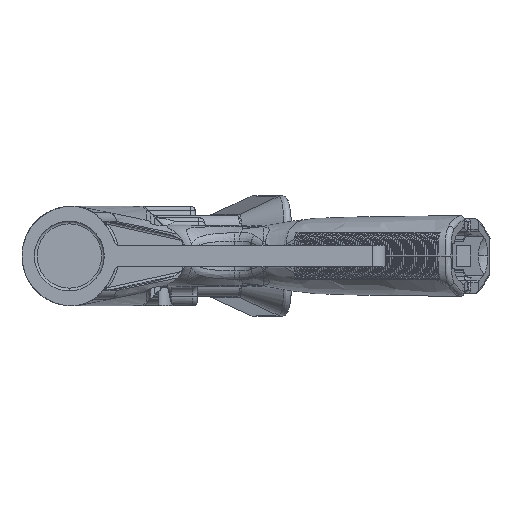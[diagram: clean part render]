
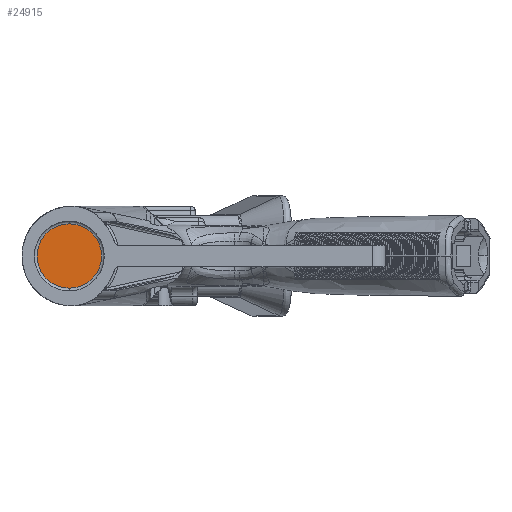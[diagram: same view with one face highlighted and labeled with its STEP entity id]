
A CAD part, left-side view. The second image highlights one B-rep face of the part: STEP entity #24915.
In plain terms, the highlighted planar face has unit normal (-1, 0, 0).
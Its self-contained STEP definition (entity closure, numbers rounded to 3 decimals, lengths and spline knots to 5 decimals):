
#762 = CIRCLE ( 'NONE', #21061, 0.47244 ) ;
#9850 = AXIS2_PLACEMENT_3D ( 'NONE', #50701, #78847, #23850 ) ;
#11358 = CIRCLE ( 'NONE', #9850, 0.47244 ) ;
#11780 = DIRECTION ( 'NONE',  ( 0., 0., 1. ) ) ;
#12661 = VERTEX_POINT ( 'NONE', #74836 ) ;
#18324 = EDGE_CURVE ( 'NONE', #82967, #12661, #11358, .T. ) ;
#21061 = AXIS2_PLACEMENT_3D ( 'NONE', #56639, #43883, #22078 ) ;
#22078 = DIRECTION ( 'NONE',  ( 0., 0., 1. ) ) ;
#23820 = ORIENTED_EDGE ( 'NONE', *, *, #65666, .T. ) ;
#23850 = DIRECTION ( 'NONE',  ( 0., 0., 1. ) ) ;
#24915 = ADVANCED_FACE ( 'NONE', ( #54492 ), #25848, .T. ) ;
#25848 = PLANE ( 'NONE',  #40679 ) ;
#39857 = EDGE_LOOP ( 'NONE', ( #60450, #23820 ) ) ;
#40679 = AXIS2_PLACEMENT_3D ( 'NONE', #46754, #80406, #11780 ) ;
#43883 = DIRECTION ( 'NONE',  ( -1., 0., 0. ) ) ;
#46754 = CARTESIAN_POINT ( 'NONE',  ( -14.68504, 0.87992, 0. ) ) ;
#50701 = CARTESIAN_POINT ( 'NONE',  ( -14.68504, 0.87992, 0. ) ) ;
#54492 = FACE_OUTER_BOUND ( 'NONE', #39857, .T. ) ;
#56639 = CARTESIAN_POINT ( 'NONE',  ( -14.68504, 0.87992, 0. ) ) ;
#60450 = ORIENTED_EDGE ( 'NONE', *, *, #18324, .T. ) ;
#65666 = EDGE_CURVE ( 'NONE', #12661, #82967, #762, .T. ) ;
#70736 = CARTESIAN_POINT ( 'NONE',  ( -14.68504, 0.87992, 0.47244 ) ) ;
#74836 = CARTESIAN_POINT ( 'NONE',  ( -14.68504, 0.87992, -0.47244 ) ) ;
#78847 = DIRECTION ( 'NONE',  ( -1., 0., 0. ) ) ;
#80406 = DIRECTION ( 'NONE',  ( -1., 0., 0. ) ) ;
#82967 = VERTEX_POINT ( 'NONE', #70736 ) ;
